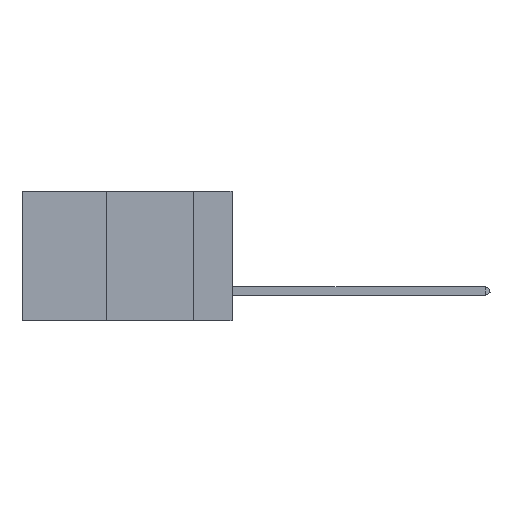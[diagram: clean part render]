
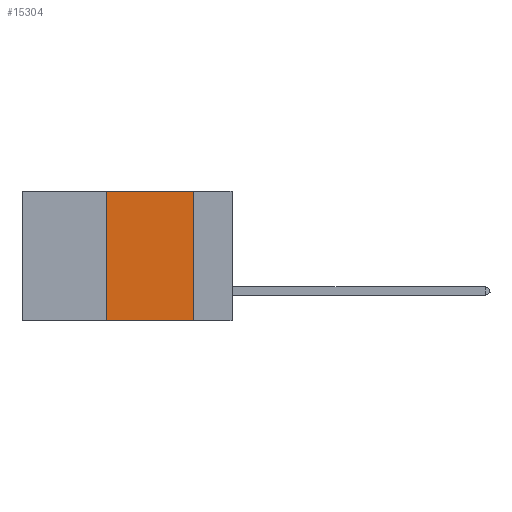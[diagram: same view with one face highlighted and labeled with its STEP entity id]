
A CAD part, left-side view. The second image highlights one B-rep face of the part: STEP entity #15304.
In plain terms, the highlighted planar face has unit normal (-1, 0, 0).
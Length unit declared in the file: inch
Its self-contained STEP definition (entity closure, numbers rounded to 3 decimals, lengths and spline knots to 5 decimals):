
#24 = EDGE_CURVE ( 'NONE', #4589, #13356, #10838, .T. ) ;
#697 = CARTESIAN_POINT ( 'NONE',  ( 0., 0.11, 0. ) ) ;
#1753 = AXIS2_PLACEMENT_3D ( 'NONE', #13650, #4799, #9171 ) ;
#3214 = DIRECTION ( 'NONE',  ( 0., 0., -1. ) ) ;
#3678 = EDGE_CURVE ( 'NONE', #14799, #4589, #18130, .T. ) ;
#4589 = VERTEX_POINT ( 'NONE', #8858 ) ;
#4649 = DIRECTION ( 'NONE',  ( 0., -1., 0. ) ) ;
#4749 = EDGE_CURVE ( 'NONE', #13356, #16333, #5830, .T. ) ;
#4799 = DIRECTION ( 'NONE',  ( 1., 0., 0. ) ) ;
#5785 = VECTOR ( 'NONE', #9832, 39.37008 ) ;
#5830 = LINE ( 'NONE', #12284, #6997 ) ;
#6642 = EDGE_CURVE ( 'NONE', #14799, #16333, #17124, .T. ) ;
#6961 = VECTOR ( 'NONE', #4649, 39.37008 ) ;
#6997 = VECTOR ( 'NONE', #3214, 39.37008 ) ;
#7275 = FACE_OUTER_BOUND ( 'NONE', #18985, .T. ) ;
#8858 = CARTESIAN_POINT ( 'NONE',  ( 0., 0.36, 0. ) ) ;
#9171 = DIRECTION ( 'NONE',  ( 0., 0., -1. ) ) ;
#9832 = DIRECTION ( 'NONE',  ( 0., -1., 0. ) ) ;
#10780 = ORIENTED_EDGE ( 'NONE', *, *, #24, .F. ) ;
#10838 = LINE ( 'NONE', #12838, #5785 ) ;
#10987 = CARTESIAN_POINT ( 'NONE',  ( 0., 0.36, -0.37 ) ) ;
#12284 = CARTESIAN_POINT ( 'NONE',  ( 0., 0.11, 0. ) ) ;
#12838 = CARTESIAN_POINT ( 'NONE',  ( 0., 0.6, 0. ) ) ;
#13356 = VERTEX_POINT ( 'NONE', #697 ) ;
#13650 = CARTESIAN_POINT ( 'NONE',  ( 0., 0.6, 0. ) ) ;
#13689 = ORIENTED_EDGE ( 'NONE', *, *, #3678, .F. ) ;
#13963 = DIRECTION ( 'NONE',  ( 0., 0., 1. ) ) ;
#14799 = VERTEX_POINT ( 'NONE', #10987 ) ;
#15304 = ADVANCED_FACE ( 'NONE', ( #7275 ), #16471, .F. ) ;
#16320 = CARTESIAN_POINT ( 'NONE',  ( 0., 0.6, -0.37 ) ) ;
#16333 = VERTEX_POINT ( 'NONE', #16542 ) ;
#16422 = ORIENTED_EDGE ( 'NONE', *, *, #4749, .F. ) ;
#16471 = PLANE ( 'NONE',  #1753 ) ;
#16542 = CARTESIAN_POINT ( 'NONE',  ( 0., 0.11, -0.37 ) ) ;
#16869 = CARTESIAN_POINT ( 'NONE',  ( 0., 0.36, 0. ) ) ;
#17124 = LINE ( 'NONE', #16320, #6961 ) ;
#17318 = ORIENTED_EDGE ( 'NONE', *, *, #6642, .T. ) ;
#18130 = LINE ( 'NONE', #16869, #18571 ) ;
#18571 = VECTOR ( 'NONE', #13963, 39.37008 ) ;
#18985 = EDGE_LOOP ( 'NONE', ( #16422, #10780, #13689, #17318 ) ) ;
